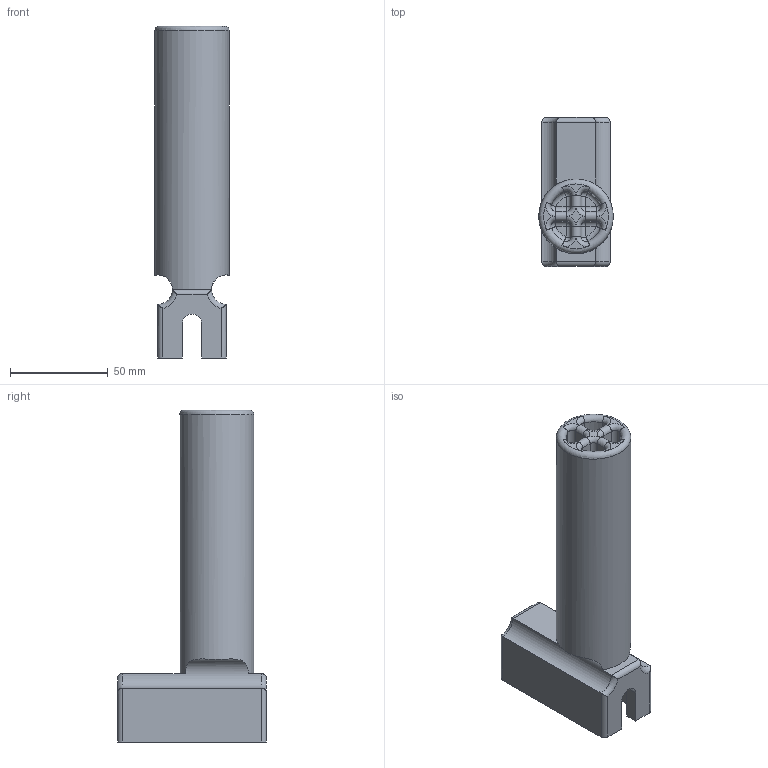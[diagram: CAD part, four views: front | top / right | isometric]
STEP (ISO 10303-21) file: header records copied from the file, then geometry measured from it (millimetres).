
FILE_DESCRIPTION (( 'STEP AP214' ), '1' );
FILE_NAME ('Trellais_Arm.step', '2016-04-19T10:44:24', ( 'WarFairy' ), ( '' ), 'SwSTEP 2.0', 'SolidWorks 2015', '' );
FILE_SCHEMA (( 'AUTOMOTIVE_DESIGN' ));
Length unit declared in the file: millimetre
Products named in the file (1): Trellais_Arm
Bounding box: 38.1 x 76.2 x 169.9 mm (x, y, z)
Volume: 148099.4 mm3; surface area: 48279.7 mm2
Topology: 1 solids, 1 shells, 102 faces, 235 edges, 123 vertices
Faces by surface type: cylinder 39, plane 30, torus 21, sphere 12
Full cylindrical faces by diameter (mm): 38.1 x1
Entity records: 2978 total; most frequent: CARTESIAN_POINT 685, DIRECTION 534, ORIENTED_EDGE 438, AXIS2_PLACEMENT_3D 222, EDGE_CURVE 219, VERTEX_POINT 121, CIRCLE 119, EDGE_LOOP 104
